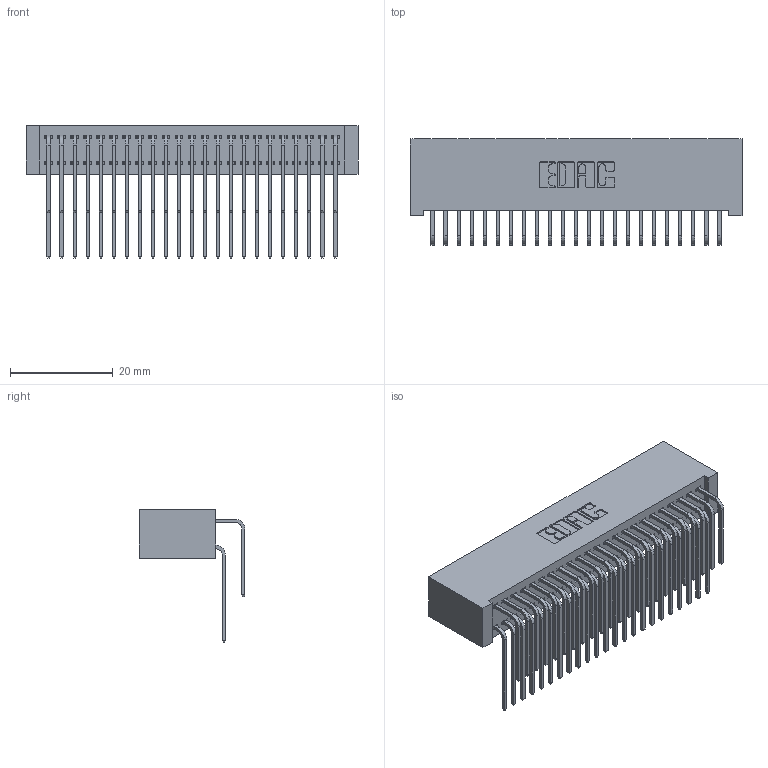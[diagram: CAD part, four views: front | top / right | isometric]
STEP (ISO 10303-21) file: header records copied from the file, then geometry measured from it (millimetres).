
FILE_DESCRIPTION (( 'STEP AP203' ), '1' );
FILE_NAME ('392-046-559-201.STEP', '2019-10-08T00:07:44', ( '' ), ( '' ), 'SwSTEP 2.0', 'SolidWorks 2016', '' );
FILE_SCHEMA (( 'CONFIG_CONTROL_DESIGN' ));
Length unit declared in the file: inch
Products named in the file (4): 345-292-001_559 Tail - 2; 392-046-559-201; 342 Part_Lugless; 345-292-001_558 559 Tail - 1
Assembly tree (47 placements, depth 2):
  392-046-559-201
    342 Part_Lugless
    345-292-001_558 559 Tail - 1  x23
    345-292-001_559 Tail - 2  x23
Bounding box: 64.67 x 20.64 x 25.78 mm (x, y, z)
Volume: 6425.4 mm3; surface area: 11637.4 mm2
Topology: 47 solids, 47 shells, 2586 faces, 7681 edges, 5058 vertices
Faces by surface type: plane 1810, cylinder 776
Entity records: 18629 total; most frequent: CARTESIAN_POINT 3157, ORIENTED_EDGE 3042, DIRECTION 2705, EDGE_CURVE 1521, VECTOR 1361, LINE 1361, VERTEX_POINT 1010, AXIS2_PLACEMENT_3D 672
